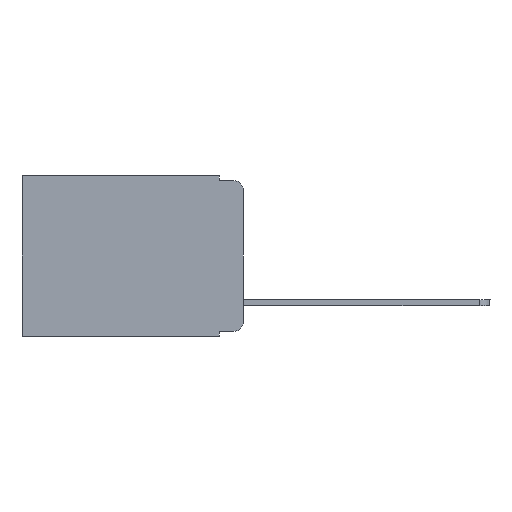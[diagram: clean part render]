
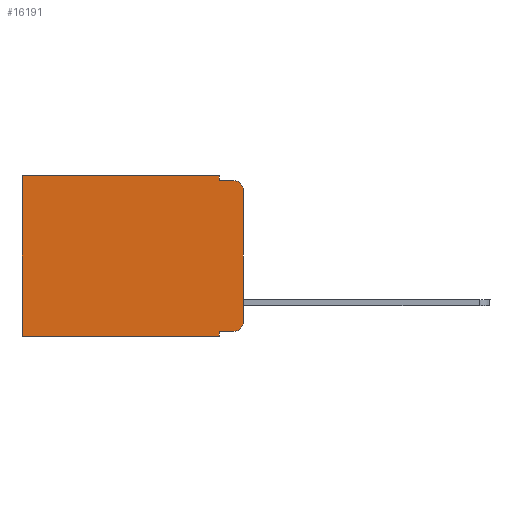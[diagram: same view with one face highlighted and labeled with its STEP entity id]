
A CAD part, left-side view. The second image highlights one B-rep face of the part: STEP entity #16191.
In plain terms, the highlighted planar face has unit normal (-1, 0, 0).
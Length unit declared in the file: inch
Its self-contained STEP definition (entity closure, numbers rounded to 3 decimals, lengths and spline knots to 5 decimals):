
#80 = EDGE_CURVE ( 'NONE', #19777, #14960, #11671, .T. ) ;
#175 = CIRCLE ( 'NONE', #15278, 0.02 ) ;
#489 = VERTEX_POINT ( 'NONE', #13925 ) ;
#801 = EDGE_CURVE ( 'NONE', #11430, #4886, #6329, .T. ) ;
#1164 = CARTESIAN_POINT ( 'NONE',  ( 0.298, 0., 0. ) ) ;
#1200 = ORIENTED_EDGE ( 'NONE', *, *, #10621, .F. ) ;
#1553 = CARTESIAN_POINT ( 'NONE',  ( 0.298, 0., -0.343 ) ) ;
#1562 = DIRECTION ( 'NONE',  ( 0., 0., -1. ) ) ;
#1808 = VERTEX_POINT ( 'NONE', #16631 ) ;
#1920 = EDGE_CURVE ( 'NONE', #18634, #3688, #8570, .T. ) ;
#1950 = CARTESIAN_POINT ( 'NONE',  ( 0.298, 0.473, -0.343 ) ) ;
#2203 = ORIENTED_EDGE ( 'NONE', *, *, #13428, .F. ) ;
#2831 = ORIENTED_EDGE ( 'NONE', *, *, #1920, .T. ) ;
#3060 = DIRECTION ( 'NONE',  ( 0., 0., -1. ) ) ;
#3311 = ORIENTED_EDGE ( 'NONE', *, *, #7165, .T. ) ;
#3388 = EDGE_CURVE ( 'NONE', #1808, #18634, #12526, .T. ) ;
#3577 = CARTESIAN_POINT ( 'NONE',  ( 0.298, 0.051, -0.01 ) ) ;
#3688 = VERTEX_POINT ( 'NONE', #1950 ) ;
#4254 = ORIENTED_EDGE ( 'NONE', *, *, #13715, .T. ) ;
#4519 = VECTOR ( 'NONE', #1562, 39.37008 ) ;
#4584 = DIRECTION ( 'NONE',  ( -1., 0., 0. ) ) ;
#4595 = ORIENTED_EDGE ( 'NONE', *, *, #11397, .F. ) ;
#4741 = ORIENTED_EDGE ( 'NONE', *, *, #80, .F. ) ;
#4886 = VERTEX_POINT ( 'NONE', #16938 ) ;
#4911 = DIRECTION ( 'NONE',  ( 0., -1., 0. ) ) ;
#6143 = DIRECTION ( 'NONE',  ( 0., 1., 0. ) ) ;
#6329 = LINE ( 'NONE', #1164, #21428 ) ;
#6553 = DIRECTION ( 'NONE',  ( 0., 0., -1. ) ) ;
#6861 = AXIS2_PLACEMENT_3D ( 'NONE', #11508, #4584, #6553 ) ;
#6987 = LINE ( 'NONE', #3577, #15418 ) ;
#7028 = CARTESIAN_POINT ( 'NONE',  ( 0.298, 0.473, 0. ) ) ;
#7165 = EDGE_CURVE ( 'NONE', #12943, #4886, #175, .T. ) ;
#7752 = ORIENTED_EDGE ( 'NONE', *, *, #3388, .T. ) ;
#8261 = ORIENTED_EDGE ( 'NONE', *, *, #20168, .T. ) ;
#8466 = CARTESIAN_POINT ( 'NONE',  ( 0.298, 0., -0.03 ) ) ;
#8570 = LINE ( 'NONE', #7028, #21306 ) ;
#8666 = DIRECTION ( 'NONE',  ( 0., 0., -1. ) ) ;
#8678 = DIRECTION ( 'NONE',  ( 0., 0., -1. ) ) ;
#9245 = CARTESIAN_POINT ( 'NONE',  ( 0.298, 0.02, -0.333 ) ) ;
#9532 = DIRECTION ( 'NONE',  ( 0., 0., -1. ) ) ;
#9931 = CARTESIAN_POINT ( 'NONE',  ( 0.298, 0.051, 0. ) ) ;
#10621 = EDGE_CURVE ( 'NONE', #16433, #489, #6987, .T. ) ;
#10642 = CARTESIAN_POINT ( 'NONE',  ( 0.298, 0.051, -0.01 ) ) ;
#10803 = ORIENTED_EDGE ( 'NONE', *, *, #801, .F. ) ;
#11093 = CARTESIAN_POINT ( 'NONE',  ( 0.298, 0., 0. ) ) ;
#11196 = PLANE ( 'NONE',  #15931 ) ;
#11397 = EDGE_CURVE ( 'NONE', #14960, #3688, #18625, .T. ) ;
#11430 = VERTEX_POINT ( 'NONE', #8466 ) ;
#11508 = CARTESIAN_POINT ( 'NONE',  ( 0.298, 0.02, -0.03 ) ) ;
#11623 = CARTESIAN_POINT ( 'NONE',  ( 0.298, 0.051, -0.343 ) ) ;
#11671 = LINE ( 'NONE', #9931, #4519 ) ;
#12328 = DIRECTION ( 'NONE',  ( 0., 0., -1. ) ) ;
#12526 = LINE ( 'NONE', #11093, #14052 ) ;
#12943 = VERTEX_POINT ( 'NONE', #9245 ) ;
#13428 = EDGE_CURVE ( 'NONE', #1808, #16433, #13840, .T. ) ;
#13715 = EDGE_CURVE ( 'NONE', #19777, #12943, #19676, .T. ) ;
#13840 = LINE ( 'NONE', #17273, #19370 ) ;
#13925 = CARTESIAN_POINT ( 'NONE',  ( 0.298, 0.02, -0.01 ) ) ;
#14052 = VECTOR ( 'NONE', #6143, 39.37008 ) ;
#14497 = DIRECTION ( 'NONE',  ( -1., 0., 0. ) ) ;
#14711 = CARTESIAN_POINT ( 'NONE',  ( 0.298, 0.051, -0.333 ) ) ;
#14960 = VERTEX_POINT ( 'NONE', #11623 ) ;
#15129 = VECTOR ( 'NONE', #4911, 39.37008 ) ;
#15278 = AXIS2_PLACEMENT_3D ( 'NONE', #18137, #14497, #3060 ) ;
#15418 = VECTOR ( 'NONE', #15460, 39.37008 ) ;
#15460 = DIRECTION ( 'NONE',  ( 0., -1., 0. ) ) ;
#15931 = AXIS2_PLACEMENT_3D ( 'NONE', #17926, #20730, #12328 ) ;
#16191 = ADVANCED_FACE ( 'NONE', ( #17814 ), #11196, .F. ) ;
#16412 = EDGE_LOOP ( 'NONE', ( #10803, #8261, #1200, #2203, #7752, #2831, #4595, #4741, #4254, #3311 ) ) ;
#16433 = VERTEX_POINT ( 'NONE', #10642 ) ;
#16631 = CARTESIAN_POINT ( 'NONE',  ( 0.298, 0.051, 0. ) ) ;
#16938 = CARTESIAN_POINT ( 'NONE',  ( 0.298, 0., -0.313 ) ) ;
#17273 = CARTESIAN_POINT ( 'NONE',  ( 0.298, 0.051, 0. ) ) ;
#17814 = FACE_OUTER_BOUND ( 'NONE', #16412, .T. ) ;
#17926 = CARTESIAN_POINT ( 'NONE',  ( 0.298, 0., 0. ) ) ;
#18137 = CARTESIAN_POINT ( 'NONE',  ( 0.298, 0.02, -0.313 ) ) ;
#18402 = DIRECTION ( 'NONE',  ( 0., 1., 0. ) ) ;
#18625 = LINE ( 'NONE', #1553, #20371 ) ;
#18634 = VERTEX_POINT ( 'NONE', #19014 ) ;
#19014 = CARTESIAN_POINT ( 'NONE',  ( 0.298, 0.473, 0. ) ) ;
#19370 = VECTOR ( 'NONE', #8666, 39.37008 ) ;
#19545 = CIRCLE ( 'NONE', #6861, 0.02 ) ;
#19676 = LINE ( 'NONE', #14711, #15129 ) ;
#19777 = VERTEX_POINT ( 'NONE', #21556 ) ;
#20168 = EDGE_CURVE ( 'NONE', #11430, #489, #19545, .T. ) ;
#20371 = VECTOR ( 'NONE', #18402, 39.37008 ) ;
#20730 = DIRECTION ( 'NONE',  ( 1., 0., 0. ) ) ;
#21306 = VECTOR ( 'NONE', #8678, 39.37008 ) ;
#21428 = VECTOR ( 'NONE', #9532, 39.37008 ) ;
#21556 = CARTESIAN_POINT ( 'NONE',  ( 0.298, 0.051, -0.333 ) ) ;
